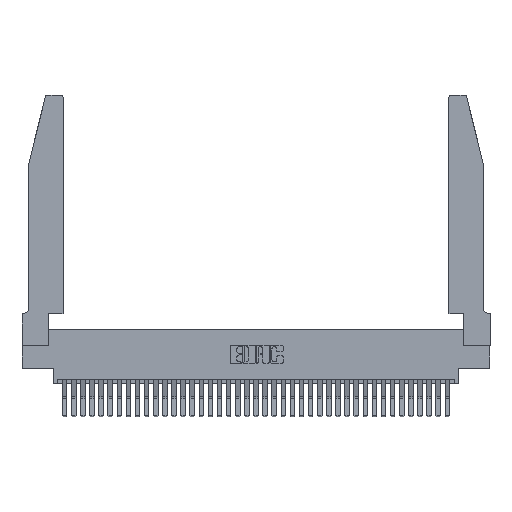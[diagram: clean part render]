
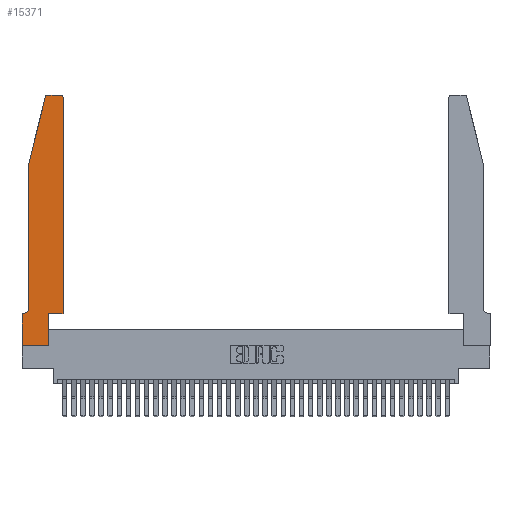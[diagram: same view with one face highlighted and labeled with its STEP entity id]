
A CAD part, top view. The second image highlights one B-rep face of the part: STEP entity #15371.
In plain terms, the highlighted planar face has unit normal (0, 0, 1).
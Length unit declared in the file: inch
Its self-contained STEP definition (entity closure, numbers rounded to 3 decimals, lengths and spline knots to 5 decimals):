
#121 = LINE ( 'NONE', #17233, #4292 ) ;
#140 = EDGE_CURVE ( 'NONE', #38412, #24256, #121, .T. ) ;
#1354 = CARTESIAN_POINT ( 'NONE',  ( 0.4205, 2.72, 0.37 ) ) ;
#1377 = DIRECTION ( 'NONE',  ( 1., 0., 0. ) ) ;
#1593 = DIRECTION ( 'NONE',  ( 0., 1., 0. ) ) ;
#1613 = LINE ( 'NONE', #9430, #16479 ) ;
#2593 = LINE ( 'NONE', #10444, #5874 ) ;
#2832 = EDGE_CURVE ( 'NONE', #3733, #8837, #26894, .T. ) ;
#3229 = CARTESIAN_POINT ( 'NONE',  ( 0., 0.35, 0.37 ) ) ;
#3431 = CARTESIAN_POINT ( 'NONE',  ( 0.2605, 2.75, 0.37 ) ) ;
#3625 = CARTESIAN_POINT ( 'NONE',  ( 0., 0., 0.37 ) ) ;
#3733 = VERTEX_POINT ( 'NONE', #35015 ) ;
#3821 = DIRECTION ( 'NONE',  ( 0., -1., 0. ) ) ;
#4292 = VECTOR ( 'NONE', #38171, 39.37008 ) ;
#4302 = CARTESIAN_POINT ( 'NONE',  ( 0.2865, 0.35, 0.37 ) ) ;
#4437 = VERTEX_POINT ( 'NONE', #11005 ) ;
#5109 = EDGE_CURVE ( 'NONE', #4437, #16277, #36671, .T. ) ;
#5155 = ORIENTED_EDGE ( 'NONE', *, *, #11730, .T. ) ;
#5413 = ORIENTED_EDGE ( 'NONE', *, *, #13495, .T. ) ;
#5874 = VECTOR ( 'NONE', #38368, 39.37008 ) ;
#6205 = EDGE_CURVE ( 'NONE', #34287, #25861, #12314, .T. ) ;
#6862 = CARTESIAN_POINT ( 'NONE',  ( 0.284, 2.72, 0.37 ) ) ;
#7438 = CARTESIAN_POINT ( 'NONE',  ( 0.0055, 0.35, 0.37 ) ) ;
#8081 = LINE ( 'NONE', #33603, #13158 ) ;
#8164 = CARTESIAN_POINT ( 'NONE',  ( 0.284, 2.75, 0.37 ) ) ;
#8517 = CARTESIAN_POINT ( 'NONE',  ( 0.0755, 2., 0.37 ) ) ;
#8837 = VERTEX_POINT ( 'NONE', #8164 ) ;
#9430 = CARTESIAN_POINT ( 'NONE',  ( 0.2865, 0.35, 0.37 ) ) ;
#9437 = DIRECTION ( 'NONE',  ( 0., 0., 1. ) ) ;
#9648 = VERTEX_POINT ( 'NONE', #29823 ) ;
#9858 = DIRECTION ( 'NONE',  ( 0., 0., 1. ) ) ;
#10444 = CARTESIAN_POINT ( 'NONE',  ( 0.4505, 0.35, 0.37 ) ) ;
#10813 = FACE_OUTER_BOUND ( 'NONE', #12107, .T. ) ;
#11005 = CARTESIAN_POINT ( 'NONE',  ( 0.25487, 2.72718, 0.37 ) ) ;
#11044 = EDGE_CURVE ( 'NONE', #24256, #9648, #38156, .T. ) ;
#11365 = ORIENTED_EDGE ( 'NONE', *, *, #11044, .T. ) ;
#11585 = ORIENTED_EDGE ( 'NONE', *, *, #140, .T. ) ;
#11730 = EDGE_CURVE ( 'NONE', #19296, #3733, #35246, .T. ) ;
#12107 = EDGE_LOOP ( 'NONE', ( #27016, #38222, #19040, #12430, #25793, #5413, #11585, #11365, #19445, #34579, #16162, #5155 ) ) ;
#12314 = CIRCLE ( 'NONE', #37438, 0.07 ) ;
#12430 = ORIENTED_EDGE ( 'NONE', *, *, #36921, .T. ) ;
#12437 = EDGE_CURVE ( 'NONE', #25923, #19296, #2593, .T. ) ;
#12498 = CARTESIAN_POINT ( 'NONE',  ( 0.0755, 2., 0.37 ) ) ;
#13158 = VECTOR ( 'NONE', #16251, 39.37008 ) ;
#13495 = EDGE_CURVE ( 'NONE', #25861, #38412, #8081, .T. ) ;
#13724 = AXIS2_PLACEMENT_3D ( 'NONE', #6862, #9858, #1377 ) ;
#14957 = DIRECTION ( 'NONE',  ( 0., 0., -1. ) ) ;
#15371 = ADVANCED_FACE ( 'NONE', ( #10813 ), #23487, .T. ) ;
#16162 = ORIENTED_EDGE ( 'NONE', *, *, #12437, .T. ) ;
#16251 = DIRECTION ( 'NONE',  ( -1., 0., 0. ) ) ;
#16277 = VERTEX_POINT ( 'NONE', #23284 ) ;
#16479 = VECTOR ( 'NONE', #1593, 39.37008 ) ;
#16978 = DIRECTION ( 'NONE',  ( 1., 0., 0. ) ) ;
#17137 = VECTOR ( 'NONE', #27029, 39.37008 ) ;
#17233 = CARTESIAN_POINT ( 'NONE',  ( 0., 0., 0.37 ) ) ;
#18181 = VECTOR ( 'NONE', #16978, 39.37008 ) ;
#18625 = DIRECTION ( 'NONE',  ( 1., 0., 0. ) ) ;
#19040 = ORIENTED_EDGE ( 'NONE', *, *, #5109, .T. ) ;
#19296 = VERTEX_POINT ( 'NONE', #19458 ) ;
#19445 = ORIENTED_EDGE ( 'NONE', *, *, #23690, .T. ) ;
#19458 = CARTESIAN_POINT ( 'NONE',  ( 0.4505, 2.72, 0.37 ) ) ;
#20269 = DIRECTION ( 'NONE',  ( -0.239, -0.971, 0. ) ) ;
#20339 = VECTOR ( 'NONE', #18625, 39.37008 ) ;
#20702 = CIRCLE ( 'NONE', #13724, 0.03 ) ;
#21317 = AXIS2_PLACEMENT_3D ( 'NONE', #3229, #9437, #33250 ) ;
#22116 = DIRECTION ( 'NONE',  ( 0., 0., 1. ) ) ;
#22876 = CARTESIAN_POINT ( 'NONE',  ( 0., 0., 0.37 ) ) ;
#23284 = CARTESIAN_POINT ( 'NONE',  ( 0.0755, 2., 0.37 ) ) ;
#23487 = PLANE ( 'NONE',  #21317 ) ;
#23582 = CARTESIAN_POINT ( 'NONE',  ( 0.0755, 0.42, 0.37 ) ) ;
#23690 = EDGE_CURVE ( 'NONE', #9648, #37302, #1613, .T. ) ;
#23825 = CARTESIAN_POINT ( 'NONE',  ( 0., 0.35, 0.37 ) ) ;
#24256 = VERTEX_POINT ( 'NONE', #3625 ) ;
#25793 = ORIENTED_EDGE ( 'NONE', *, *, #6205, .T. ) ;
#25861 = VERTEX_POINT ( 'NONE', #7438 ) ;
#25923 = VERTEX_POINT ( 'NONE', #30876 ) ;
#26881 = DIRECTION ( 'NONE',  ( -1., 0., 0. ) ) ;
#26894 = LINE ( 'NONE', #3431, #17137 ) ;
#27016 = ORIENTED_EDGE ( 'NONE', *, *, #2832, .T. ) ;
#27029 = DIRECTION ( 'NONE',  ( -1., 0., 0. ) ) ;
#27779 = VECTOR ( 'NONE', #3821, 39.37008 ) ;
#27794 = CARTESIAN_POINT ( 'NONE',  ( 0.0055, 0.42, 0.37 ) ) ;
#29823 = CARTESIAN_POINT ( 'NONE',  ( 0.2865, 0., 0.37 ) ) ;
#30852 = LINE ( 'NONE', #38173, #18181 ) ;
#30876 = CARTESIAN_POINT ( 'NONE',  ( 0.4505, 0.35, 0.37 ) ) ;
#32048 = LINE ( 'NONE', #12498, #27779 ) ;
#33250 = DIRECTION ( 'NONE',  ( 1., 0., 0. ) ) ;
#33497 = EDGE_CURVE ( 'NONE', #37302, #25923, #30852, .T. ) ;
#33603 = CARTESIAN_POINT ( 'NONE',  ( 0.0755, 0.35, 0.37 ) ) ;
#34287 = VERTEX_POINT ( 'NONE', #23582 ) ;
#34579 = ORIENTED_EDGE ( 'NONE', *, *, #33497, .T. ) ;
#34800 = AXIS2_PLACEMENT_3D ( 'NONE', #1354, #22116, #36800 ) ;
#35015 = CARTESIAN_POINT ( 'NONE',  ( 0.4205, 2.75, 0.37 ) ) ;
#35246 = CIRCLE ( 'NONE', #34800, 0.03 ) ;
#35737 = VECTOR ( 'NONE', #20269, 39.37008 ) ;
#36671 = LINE ( 'NONE', #8517, #35737 ) ;
#36800 = DIRECTION ( 'NONE',  ( 1., 0., 0. ) ) ;
#36921 = EDGE_CURVE ( 'NONE', #16277, #34287, #32048, .T. ) ;
#37302 = VERTEX_POINT ( 'NONE', #4302 ) ;
#37438 = AXIS2_PLACEMENT_3D ( 'NONE', #27794, #14957, #26881 ) ;
#37951 = EDGE_CURVE ( 'NONE', #8837, #4437, #20702, .T. ) ;
#38156 = LINE ( 'NONE', #22876, #20339 ) ;
#38171 = DIRECTION ( 'NONE',  ( 0., -1., 0. ) ) ;
#38173 = CARTESIAN_POINT ( 'NONE',  ( 0.4505, 0.35, 0.37 ) ) ;
#38222 = ORIENTED_EDGE ( 'NONE', *, *, #37951, .T. ) ;
#38368 = DIRECTION ( 'NONE',  ( 0., 1., 0. ) ) ;
#38412 = VERTEX_POINT ( 'NONE', #23825 ) ;
